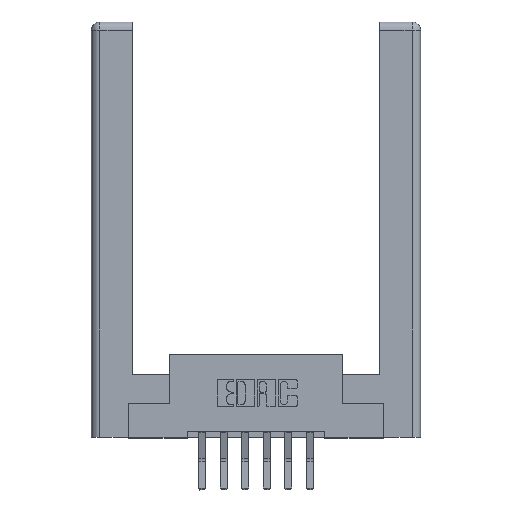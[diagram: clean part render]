
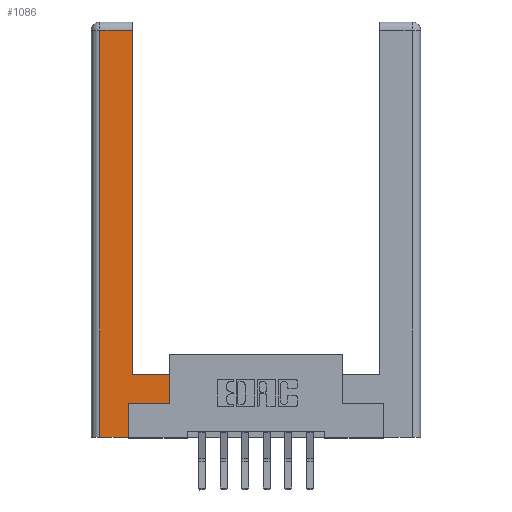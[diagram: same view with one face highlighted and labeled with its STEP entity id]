
A CAD part, top view. The second image highlights one B-rep face of the part: STEP entity #1086.
In plain terms, the highlighted planar face has unit normal (0, 0, 1).
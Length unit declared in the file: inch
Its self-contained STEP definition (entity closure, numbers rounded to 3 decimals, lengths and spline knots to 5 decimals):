
#389 = VECTOR ( 'NONE', #4389, 39.37008 ) ;
#616 = CARTESIAN_POINT ( 'NONE',  ( 0.265, 0., 0. ) ) ;
#689 = LINE ( 'NONE', #6712, #6290 ) ;
#735 = DIRECTION ( 'NONE',  ( -1., 0., 0. ) ) ;
#1086 = ADVANCED_FACE ( 'NONE', ( #6194 ), #8031, .F. ) ;
#1663 = VERTEX_POINT ( 'NONE', #2823 ) ;
#1738 = CARTESIAN_POINT ( 'NONE',  ( 0.565, 0.45, 0. ) ) ;
#1995 = ORIENTED_EDGE ( 'NONE', *, *, #4939, .T. ) ;
#2274 = ORIENTED_EDGE ( 'NONE', *, *, #4113, .T. ) ;
#2328 = EDGE_CURVE ( 'NONE', #7698, #6930, #3893, .T. ) ;
#2419 = ORIENTED_EDGE ( 'NONE', *, *, #2974, .T. ) ;
#2426 = EDGE_CURVE ( 'NONE', #8468, #8405, #6614, .T. ) ;
#2823 = CARTESIAN_POINT ( 'NONE',  ( 0.0615, 2.94, 0. ) ) ;
#2974 = EDGE_CURVE ( 'NONE', #1663, #9828, #9545, .T. ) ;
#3019 = ORIENTED_EDGE ( 'NONE', *, *, #2328, .T. ) ;
#3809 = DIRECTION ( 'NONE',  ( 0., 1., 0. ) ) ;
#3882 = VECTOR ( 'NONE', #11258, 39.37008 ) ;
#3893 = LINE ( 'NONE', #7475, #5045 ) ;
#3982 = VECTOR ( 'NONE', #11736, 39.37008 ) ;
#4113 = EDGE_CURVE ( 'NONE', #6930, #8468, #8038, .T. ) ;
#4171 = EDGE_CURVE ( 'NONE', #7075, #7568, #689, .T. ) ;
#4389 = DIRECTION ( 'NONE',  ( 1., 0., 0. ) ) ;
#4429 = EDGE_CURVE ( 'NONE', #7568, #7698, #8483, .T. ) ;
#4939 = EDGE_CURVE ( 'NONE', #8405, #1663, #9083, .T. ) ;
#5045 = VECTOR ( 'NONE', #3809, 39.37008 ) ;
#5195 = CARTESIAN_POINT ( 'NONE',  ( 0.295, 3., 0. ) ) ;
#5441 = ORIENTED_EDGE ( 'NONE', *, *, #4171, .T. ) ;
#5887 = EDGE_CURVE ( 'NONE', #9828, #7075, #5967, .T. ) ;
#5901 = VECTOR ( 'NONE', #9839, 39.37008 ) ;
#5967 = LINE ( 'NONE', #616, #3982 ) ;
#6194 = FACE_OUTER_BOUND ( 'NONE', #7007, .T. ) ;
#6290 = VECTOR ( 'NONE', #7678, 39.37008 ) ;
#6582 = CARTESIAN_POINT ( 'NONE',  ( 0.0615, 0., 0. ) ) ;
#6614 = LINE ( 'NONE', #5195, #5901 ) ;
#6712 = CARTESIAN_POINT ( 'NONE',  ( 0.265, 0.245, 0. ) ) ;
#6930 = VERTEX_POINT ( 'NONE', #1738 ) ;
#7007 = EDGE_LOOP ( 'NONE', ( #9259, #1995, #2419, #11074, #5441, #7772, #3019, #2274 ) ) ;
#7015 = DIRECTION ( 'NONE',  ( 0., 0., -1. ) ) ;
#7075 = VERTEX_POINT ( 'NONE', #11216 ) ;
#7096 = CARTESIAN_POINT ( 'NONE',  ( 0.295, 2.94, 0. ) ) ;
#7254 = CARTESIAN_POINT ( 'NONE',  ( 0.565, 0.245, 0. ) ) ;
#7475 = CARTESIAN_POINT ( 'NONE',  ( 0.565, 0.45, 0. ) ) ;
#7568 = VERTEX_POINT ( 'NONE', #9135 ) ;
#7678 = DIRECTION ( 'NONE',  ( 0., 1., 0. ) ) ;
#7698 = VERTEX_POINT ( 'NONE', #8393 ) ;
#7772 = ORIENTED_EDGE ( 'NONE', *, *, #4429, .T. ) ;
#8031 = PLANE ( 'NONE',  #10157 ) ;
#8038 = LINE ( 'NONE', #9256, #11731 ) ;
#8203 = CARTESIAN_POINT ( 'NONE',  ( 0.295, 0.45, 0. ) ) ;
#8393 = CARTESIAN_POINT ( 'NONE',  ( 0.565, 0.245, 0. ) ) ;
#8405 = VERTEX_POINT ( 'NONE', #7096 ) ;
#8468 = VERTEX_POINT ( 'NONE', #8203 ) ;
#8483 = LINE ( 'NONE', #7254, #389 ) ;
#9083 = LINE ( 'NONE', #11499, #11724 ) ;
#9135 = CARTESIAN_POINT ( 'NONE',  ( 0.265, 0.245, 0. ) ) ;
#9256 = CARTESIAN_POINT ( 'NONE',  ( 0.295, 0.45, 0. ) ) ;
#9259 = ORIENTED_EDGE ( 'NONE', *, *, #2426, .T. ) ;
#9352 = CARTESIAN_POINT ( 'NONE',  ( 0.0615, 0., 0. ) ) ;
#9545 = LINE ( 'NONE', #9352, #3882 ) ;
#9828 = VERTEX_POINT ( 'NONE', #6582 ) ;
#9839 = DIRECTION ( 'NONE',  ( 0., 1., 0. ) ) ;
#10157 = AXIS2_PLACEMENT_3D ( 'NONE', #10885, #7015, #735 ) ;
#10447 = DIRECTION ( 'NONE',  ( -1., 0., 0. ) ) ;
#10885 = CARTESIAN_POINT ( 'NONE',  ( 0., 0., 0. ) ) ;
#11074 = ORIENTED_EDGE ( 'NONE', *, *, #5887, .T. ) ;
#11194 = DIRECTION ( 'NONE',  ( -1., 0., 0. ) ) ;
#11216 = CARTESIAN_POINT ( 'NONE',  ( 0.265, 0., 0. ) ) ;
#11258 = DIRECTION ( 'NONE',  ( 0., -1., 0. ) ) ;
#11499 = CARTESIAN_POINT ( 'NONE',  ( 0.0615, 2.94, 0. ) ) ;
#11724 = VECTOR ( 'NONE', #10447, 39.37008 ) ;
#11731 = VECTOR ( 'NONE', #11194, 39.37008 ) ;
#11736 = DIRECTION ( 'NONE',  ( 1., 0., 0. ) ) ;
